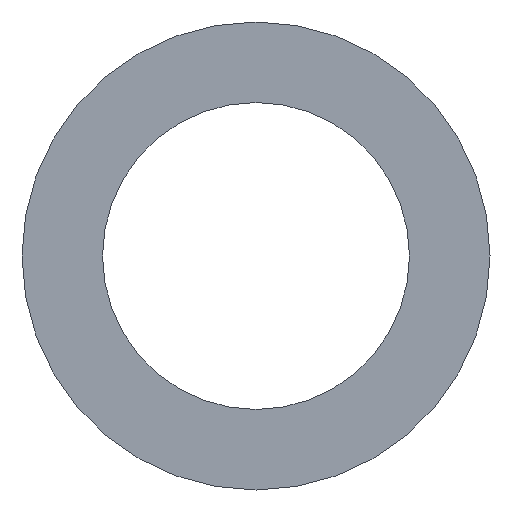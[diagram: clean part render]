
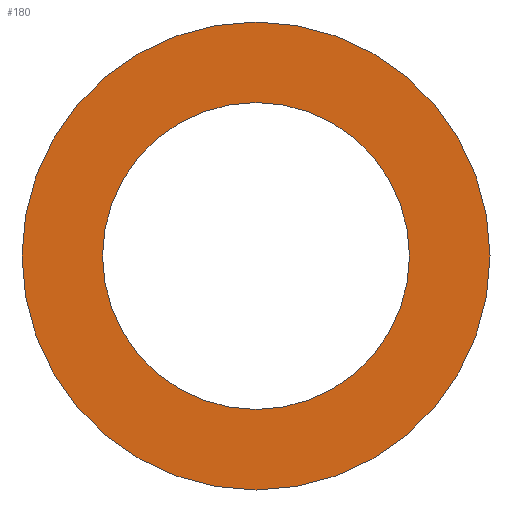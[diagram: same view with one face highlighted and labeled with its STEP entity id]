
A CAD part, front view. The second image highlights one B-rep face of the part: STEP entity #180.
In plain terms, the highlighted planar face has unit normal (0, -1, 0).
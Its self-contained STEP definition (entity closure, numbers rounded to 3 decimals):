
#15 = DIRECTION ( 'NONE',  ( 0., 1., 0. ) ) ;
#21 = DIRECTION ( 'NONE',  ( 0., 0., 1. ) ) ;
#28 = EDGE_CURVE ( 'NONE', #206, #183, #160, .T. ) ;
#35 = DIRECTION ( 'NONE',  ( 0., 1., 0. ) ) ;
#36 = DIRECTION ( 'NONE',  ( 0., 1., 0. ) ) ;
#46 = CARTESIAN_POINT ( 'NONE',  ( 0., 0., 0. ) ) ;
#47 = CIRCLE ( 'NONE', #240, 3.81 ) ;
#55 = CARTESIAN_POINT ( 'NONE',  ( 0., 0., -3.81 ) ) ;
#56 = FACE_BOUND ( 'NONE', #244, .T. ) ;
#59 = CARTESIAN_POINT ( 'NONE',  ( 0., 0., 0. ) ) ;
#60 = CIRCLE ( 'NONE', #95, 5.81 ) ;
#64 = EDGE_CURVE ( 'NONE', #97, #87, #60, .T. ) ;
#80 = CARTESIAN_POINT ( 'NONE',  ( 0., 0., 3.81 ) ) ;
#82 = CIRCLE ( 'NONE', #157, 5.81 ) ;
#87 = VERTEX_POINT ( 'NONE', #108 ) ;
#88 = EDGE_CURVE ( 'NONE', #87, #97, #82, .T. ) ;
#89 = ORIENTED_EDGE ( 'NONE', *, *, #64, .F. ) ;
#91 = DIRECTION ( 'NONE',  ( 0., 0., 1. ) ) ;
#92 = EDGE_LOOP ( 'NONE', ( #89, #188 ) ) ;
#95 = AXIS2_PLACEMENT_3D ( 'NONE', #209, #154, #91 ) ;
#97 = VERTEX_POINT ( 'NONE', #207 ) ;
#100 = AXIS2_PLACEMENT_3D ( 'NONE', #171, #36, #229 ) ;
#102 = FACE_OUTER_BOUND ( 'NONE', #92, .T. ) ;
#108 = CARTESIAN_POINT ( 'NONE',  ( 0., 0., 5.81 ) ) ;
#124 = AXIS2_PLACEMENT_3D ( 'NONE', #59, #35, #193 ) ;
#129 = ORIENTED_EDGE ( 'NONE', *, *, #28, .T. ) ;
#139 = ORIENTED_EDGE ( 'NONE', *, *, #249, .T. ) ;
#151 = CARTESIAN_POINT ( 'NONE',  ( 0., 0., 0. ) ) ;
#154 = DIRECTION ( 'NONE',  ( 0., 1., 0. ) ) ;
#157 = AXIS2_PLACEMENT_3D ( 'NONE', #151, #15, #226 ) ;
#160 = CIRCLE ( 'NONE', #100, 3.81 ) ;
#171 = CARTESIAN_POINT ( 'NONE',  ( 0., 0., 0. ) ) ;
#174 = PLANE ( 'NONE',  #124 ) ;
#180 = ADVANCED_FACE ( 'NONE', ( #102, #56 ), #174, .F. ) ;
#183 = VERTEX_POINT ( 'NONE', #80 ) ;
#188 = ORIENTED_EDGE ( 'NONE', *, *, #88, .F. ) ;
#193 = DIRECTION ( 'NONE',  ( 0., 0., 1. ) ) ;
#206 = VERTEX_POINT ( 'NONE', #55 ) ;
#207 = CARTESIAN_POINT ( 'NONE',  ( 0., 0., -5.81 ) ) ;
#209 = CARTESIAN_POINT ( 'NONE',  ( 0., 0., 0. ) ) ;
#210 = DIRECTION ( 'NONE',  ( 0., 1., 0. ) ) ;
#226 = DIRECTION ( 'NONE',  ( 0., 0., 1. ) ) ;
#229 = DIRECTION ( 'NONE',  ( 0., 0., 1. ) ) ;
#240 = AXIS2_PLACEMENT_3D ( 'NONE', #46, #210, #21 ) ;
#244 = EDGE_LOOP ( 'NONE', ( #129, #139 ) ) ;
#249 = EDGE_CURVE ( 'NONE', #183, #206, #47, .T. ) ;
